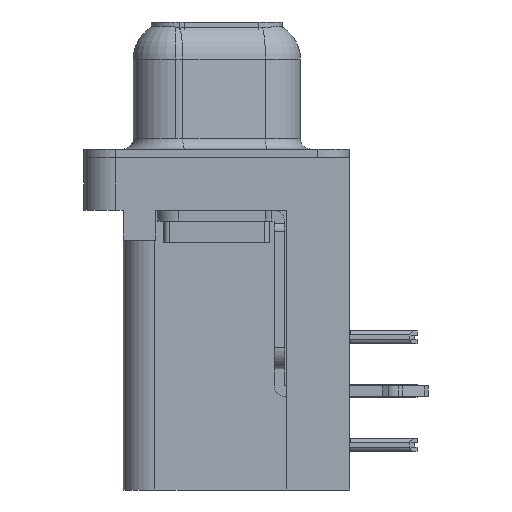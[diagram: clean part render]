
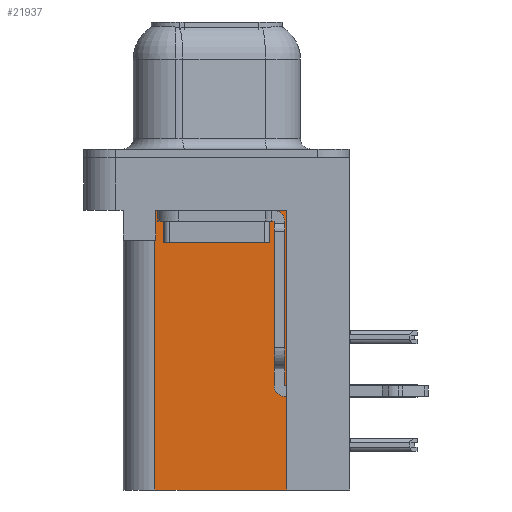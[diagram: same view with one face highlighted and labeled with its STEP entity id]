
A CAD part, left-side view. The second image highlights one B-rep face of the part: STEP entity #21937.
In plain terms, the highlighted planar face has unit normal (-1, 0, 0).
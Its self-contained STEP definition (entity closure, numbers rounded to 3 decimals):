
#181 = VECTOR ( 'NONE', #12413, 1000. ) ;
#197 = ORIENTED_EDGE ( 'NONE', *, *, #6043, .T. ) ;
#311 = LINE ( 'NONE', #32375, #181 ) ;
#2434 = CARTESIAN_POINT ( 'NONE',  ( 3.765, -3.295, -15.7 ) ) ;
#3348 = ORIENTED_EDGE ( 'NONE', *, *, #29628, .F. ) ;
#4601 = CARTESIAN_POINT ( 'NONE',  ( 3.765, 2.925, -3.9 ) ) ;
#5392 = CARTESIAN_POINT ( 'NONE',  ( 3.765, 0., -3.9 ) ) ;
#5671 = DIRECTION ( 'NONE',  ( 0., 0., -1. ) ) ;
#6043 = EDGE_CURVE ( 'NONE', #7947, #27175, #21878, .T. ) ;
#6426 = CARTESIAN_POINT ( 'NONE',  ( 3.765, -3.295, -2.5 ) ) ;
#6586 = CARTESIAN_POINT ( 'NONE',  ( 3.765, -3.295, -2.5 ) ) ;
#7251 = VERTEX_POINT ( 'NONE', #33655 ) ;
#7596 = FACE_OUTER_BOUND ( 'NONE', #21034, .T. ) ;
#7759 = VECTOR ( 'NONE', #13331, 1000. ) ;
#7764 = CARTESIAN_POINT ( 'NONE',  ( 3.765, -3.295, -15.7 ) ) ;
#7856 = LINE ( 'NONE', #10600, #7759 ) ;
#7947 = VERTEX_POINT ( 'NONE', #6586 ) ;
#8055 = VERTEX_POINT ( 'NONE', #30323 ) ;
#8162 = ORIENTED_EDGE ( 'NONE', *, *, #9021, .T. ) ;
#8379 = EDGE_CURVE ( 'NONE', #27175, #7251, #35744, .T. ) ;
#9021 = EDGE_CURVE ( 'NONE', #7251, #36702, #32282, .T. ) ;
#10600 = CARTESIAN_POINT ( 'NONE',  ( 3.765, 2.925, -15.7 ) ) ;
#11957 = DIRECTION ( 'NONE',  ( 1., 0., 0. ) ) ;
#12413 = DIRECTION ( 'NONE',  ( 0., 1., 0. ) ) ;
#13331 = DIRECTION ( 'NONE',  ( 0., 0., 1. ) ) ;
#14698 = VERTEX_POINT ( 'NONE', #7764 ) ;
#17975 = CARTESIAN_POINT ( 'NONE',  ( 3.765, 2.895, -2.5 ) ) ;
#20513 = PLANE ( 'NONE',  #23206 ) ;
#21034 = EDGE_LOOP ( 'NONE', ( #197, #29743, #8162, #3348, #25606, #35190 ) ) ;
#21453 = VECTOR ( 'NONE', #29293, 1000. ) ;
#21878 = LINE ( 'NONE', #6426, #21453 ) ;
#21937 = ADVANCED_FACE ( 'NONE', ( #7596 ), #20513, .F. ) ;
#22802 = CARTESIAN_POINT ( 'NONE',  ( 3.765, 2.895, -3.9 ) ) ;
#23206 = AXIS2_PLACEMENT_3D ( 'NONE', #29083, #11957, #31944 ) ;
#25606 = ORIENTED_EDGE ( 'NONE', *, *, #30958, .F. ) ;
#25627 = DIRECTION ( 'NONE',  ( 0., 1., 0. ) ) ;
#27175 = VERTEX_POINT ( 'NONE', #17975 ) ;
#28103 = DIRECTION ( 'NONE',  ( 0., 0., 1. ) ) ;
#29083 = CARTESIAN_POINT ( 'NONE',  ( 3.765, -3.295, -15.7 ) ) ;
#29293 = DIRECTION ( 'NONE',  ( 0., 1., 0. ) ) ;
#29628 = EDGE_CURVE ( 'NONE', #8055, #36702, #7856, .T. ) ;
#29743 = ORIENTED_EDGE ( 'NONE', *, *, #8379, .T. ) ;
#30323 = CARTESIAN_POINT ( 'NONE',  ( 3.765, 2.925, -15.7 ) ) ;
#30958 = EDGE_CURVE ( 'NONE', #14698, #8055, #311, .T. ) ;
#31552 = EDGE_CURVE ( 'NONE', #14698, #7947, #32702, .T. ) ;
#31944 = DIRECTION ( 'NONE',  ( 0., 1., 0. ) ) ;
#32282 = LINE ( 'NONE', #5392, #32319 ) ;
#32319 = VECTOR ( 'NONE', #25627, 1000. ) ;
#32375 = CARTESIAN_POINT ( 'NONE',  ( 3.765, -3.295, -15.7 ) ) ;
#32455 = VECTOR ( 'NONE', #28103, 1000. ) ;
#32702 = LINE ( 'NONE', #2434, #32455 ) ;
#33655 = CARTESIAN_POINT ( 'NONE',  ( 3.765, 2.895, -3.9 ) ) ;
#35190 = ORIENTED_EDGE ( 'NONE', *, *, #31552, .T. ) ;
#35519 = VECTOR ( 'NONE', #5671, 1000. ) ;
#35744 = LINE ( 'NONE', #22802, #35519 ) ;
#36702 = VERTEX_POINT ( 'NONE', #4601 ) ;
